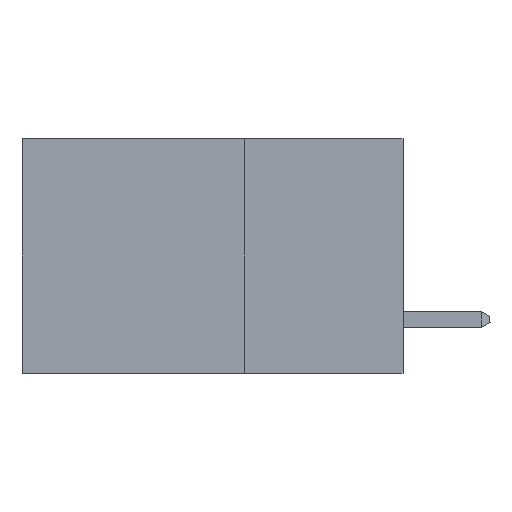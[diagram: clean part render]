
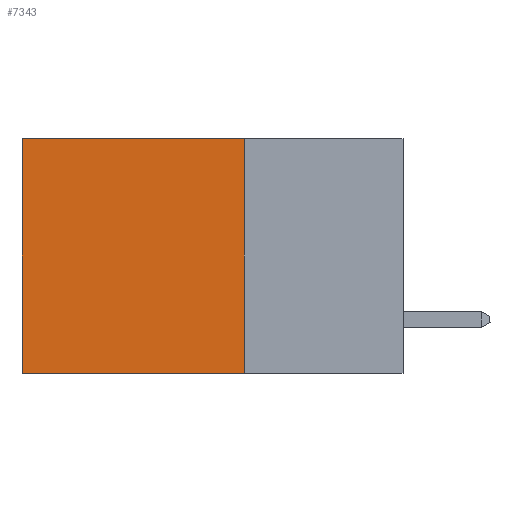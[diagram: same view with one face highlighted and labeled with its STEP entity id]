
A CAD part, left-side view. The second image highlights one B-rep face of the part: STEP entity #7343.
In plain terms, the highlighted planar face has unit normal (-1, 0, 0).
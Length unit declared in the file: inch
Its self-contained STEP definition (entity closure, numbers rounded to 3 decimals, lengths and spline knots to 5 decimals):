
#54 = DIRECTION ( 'NONE',  ( 0., 1., 0. ) ) ;
#494 = LINE ( 'NONE', #2693, #7230 ) ;
#634 = CARTESIAN_POINT ( 'NONE',  ( 0.2875, 0.25, -0.37 ) ) ;
#982 = VERTEX_POINT ( 'NONE', #2483 ) ;
#1426 = DIRECTION ( 'NONE',  ( 0., 0., -1. ) ) ;
#1604 = CARTESIAN_POINT ( 'NONE',  ( 0.2875, 0.25, 0. ) ) ;
#1712 = FACE_OUTER_BOUND ( 'NONE', #6870, .T. ) ;
#1803 = EDGE_CURVE ( 'NONE', #8247, #2689, #5592, .T. ) ;
#2136 = ORIENTED_EDGE ( 'NONE', *, *, #10037, .F. ) ;
#2174 = ORIENTED_EDGE ( 'NONE', *, *, #5103, .T. ) ;
#2483 = CARTESIAN_POINT ( 'NONE',  ( 0.2875, 0.6, 0. ) ) ;
#2629 = CARTESIAN_POINT ( 'NONE',  ( 0.2875, 0.25, 0. ) ) ;
#2689 = VERTEX_POINT ( 'NONE', #6332 ) ;
#2693 = CARTESIAN_POINT ( 'NONE',  ( 0.2875, 0.6, 0. ) ) ;
#3317 = AXIS2_PLACEMENT_3D ( 'NONE', #5783, #10181, #1426 ) ;
#4430 = DIRECTION ( 'NONE',  ( 0., 0., -1. ) ) ;
#5103 = EDGE_CURVE ( 'NONE', #8247, #982, #7935, .T. ) ;
#5518 = VECTOR ( 'NONE', #54, 39.37008 ) ;
#5592 = LINE ( 'NONE', #1604, #6939 ) ;
#5783 = CARTESIAN_POINT ( 'NONE',  ( 0.2875, 0.25, 0. ) ) ;
#5879 = LINE ( 'NONE', #634, #6009 ) ;
#6009 = VECTOR ( 'NONE', #6647, 39.37008 ) ;
#6183 = VERTEX_POINT ( 'NONE', #9401 ) ;
#6332 = CARTESIAN_POINT ( 'NONE',  ( 0.2875, 0.25, -0.37 ) ) ;
#6399 = EDGE_CURVE ( 'NONE', #982, #6183, #494, .T. ) ;
#6645 = PLANE ( 'NONE',  #3317 ) ;
#6647 = DIRECTION ( 'NONE',  ( 0., 1., 0. ) ) ;
#6870 = EDGE_LOOP ( 'NONE', ( #10207, #2136, #8172, #2174 ) ) ;
#6939 = VECTOR ( 'NONE', #7468, 39.37008 ) ;
#7230 = VECTOR ( 'NONE', #4430, 39.37008 ) ;
#7343 = ADVANCED_FACE ( 'NONE', ( #1712 ), #6645, .F. ) ;
#7429 = CARTESIAN_POINT ( 'NONE',  ( 0.2875, 0.25, 0. ) ) ;
#7468 = DIRECTION ( 'NONE',  ( 0., 0., -1. ) ) ;
#7935 = LINE ( 'NONE', #2629, #5518 ) ;
#8172 = ORIENTED_EDGE ( 'NONE', *, *, #1803, .F. ) ;
#8247 = VERTEX_POINT ( 'NONE', #7429 ) ;
#9401 = CARTESIAN_POINT ( 'NONE',  ( 0.2875, 0.6, -0.37 ) ) ;
#10037 = EDGE_CURVE ( 'NONE', #2689, #6183, #5879, .T. ) ;
#10181 = DIRECTION ( 'NONE',  ( 1., 0., 0. ) ) ;
#10207 = ORIENTED_EDGE ( 'NONE', *, *, #6399, .T. ) ;
